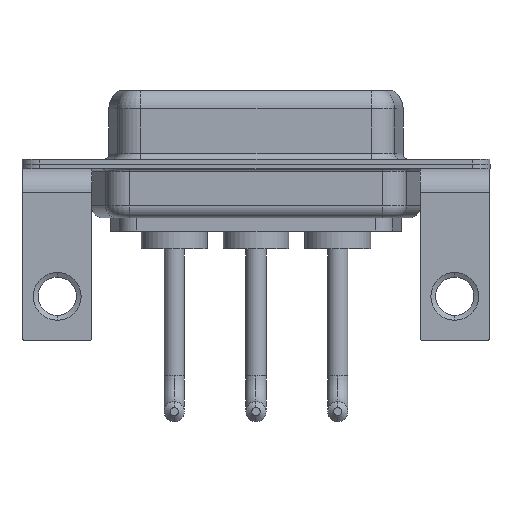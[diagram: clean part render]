
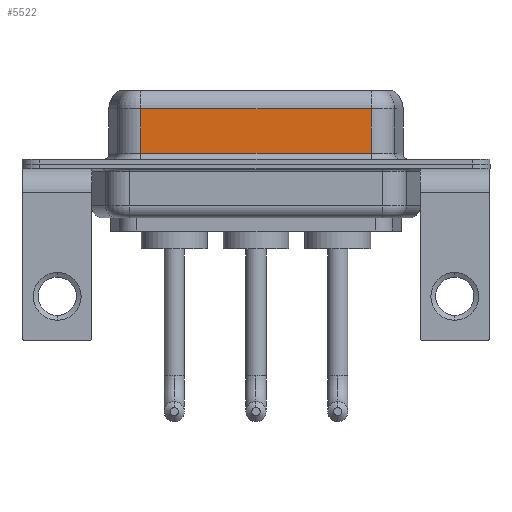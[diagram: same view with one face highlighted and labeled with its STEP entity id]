
A CAD part, front view. The second image highlights one B-rep face of the part: STEP entity #5522.
In plain terms, the highlighted planar face has unit normal (0, -1, 0).
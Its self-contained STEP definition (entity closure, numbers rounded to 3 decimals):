
#516 = DIRECTION ( 'NONE',  ( 0., 0., -1. ) ) ;
#614 = EDGE_LOOP ( 'NONE', ( #7671, #7932, #6899, #5305 ) ) ;
#710 = VERTEX_POINT ( 'NONE', #8658 ) ;
#745 = DIRECTION ( 'NONE',  ( 0., 1., 0. ) ) ;
#943 = VERTEX_POINT ( 'NONE', #5508 ) ;
#1499 = CARTESIAN_POINT ( 'NONE',  ( 26.287, -3.95, 6.4 ) ) ;
#1689 = LINE ( 'NONE', #1499, #11551 ) ;
#1693 = LINE ( 'NONE', #4755, #2042 ) ;
#1808 = EDGE_CURVE ( 'NONE', #710, #7375, #8067, .T. ) ;
#2042 = VECTOR ( 'NONE', #8696, 1000. ) ;
#2355 = LINE ( 'NONE', #8556, #7850 ) ;
#3846 = EDGE_CURVE ( 'NONE', #710, #4244, #1689, .T. ) ;
#4244 = VERTEX_POINT ( 'NONE', #8350 ) ;
#4479 = VECTOR ( 'NONE', #11188, 1000. ) ;
#4583 = CARTESIAN_POINT ( 'NONE',  ( 7.013, -3.95, 4.65 ) ) ;
#4755 = CARTESIAN_POINT ( 'NONE',  ( 26.287, -3.95, 0.9 ) ) ;
#4785 = FACE_OUTER_BOUND ( 'NONE', #614, .T. ) ;
#5305 = ORIENTED_EDGE ( 'NONE', *, *, #6521, .T. ) ;
#5508 = CARTESIAN_POINT ( 'NONE',  ( 7.013, -3.95, 0.9 ) ) ;
#5522 = ADVANCED_FACE ( 'NONE', ( #4785 ), #6787, .F. ) ;
#5759 = DIRECTION ( 'NONE',  ( 0., 0., -1. ) ) ;
#6521 = EDGE_CURVE ( 'NONE', #943, #4244, #1693, .T. ) ;
#6787 = PLANE ( 'NONE',  #8842 ) ;
#6899 = ORIENTED_EDGE ( 'NONE', *, *, #8818, .T. ) ;
#7074 = CARTESIAN_POINT ( 'NONE',  ( 26.287, -3.95, 4.65 ) ) ;
#7375 = VERTEX_POINT ( 'NONE', #4583 ) ;
#7671 = ORIENTED_EDGE ( 'NONE', *, *, #3846, .F. ) ;
#7850 = VECTOR ( 'NONE', #516, 1000. ) ;
#7932 = ORIENTED_EDGE ( 'NONE', *, *, #1808, .T. ) ;
#8067 = LINE ( 'NONE', #7074, #4479 ) ;
#8350 = CARTESIAN_POINT ( 'NONE',  ( 26.287, -3.95, 0.9 ) ) ;
#8556 = CARTESIAN_POINT ( 'NONE',  ( 7.013, -3.95, 6.4 ) ) ;
#8658 = CARTESIAN_POINT ( 'NONE',  ( 26.287, -3.95, 4.65 ) ) ;
#8696 = DIRECTION ( 'NONE',  ( 1., 0., 0. ) ) ;
#8818 = EDGE_CURVE ( 'NONE', #7375, #943, #2355, .T. ) ;
#8842 = AXIS2_PLACEMENT_3D ( 'NONE', #11837, #745, #8863 ) ;
#8863 = DIRECTION ( 'NONE',  ( 0., 0., 1. ) ) ;
#11188 = DIRECTION ( 'NONE',  ( -1., 0., 0. ) ) ;
#11551 = VECTOR ( 'NONE', #5759, 1000. ) ;
#11837 = CARTESIAN_POINT ( 'NONE',  ( 26.287, -3.95, 6.4 ) ) ;
